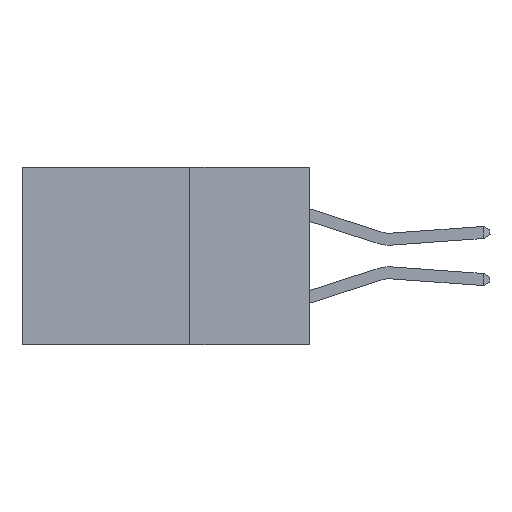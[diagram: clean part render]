
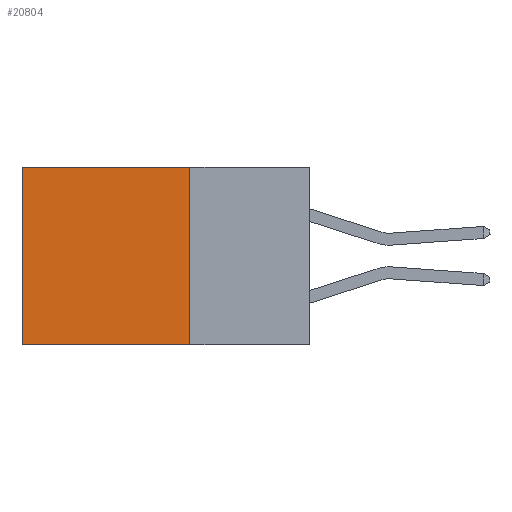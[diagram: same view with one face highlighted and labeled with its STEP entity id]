
A CAD part, left-side view. The second image highlights one B-rep face of the part: STEP entity #20804.
In plain terms, the highlighted planar face has unit normal (-1, 0, 0).
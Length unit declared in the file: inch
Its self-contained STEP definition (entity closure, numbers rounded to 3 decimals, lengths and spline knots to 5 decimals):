
#296 = EDGE_CURVE ( 'NONE', #18656, #12175, #3849, .T. ) ;
#745 = DIRECTION ( 'NONE',  ( 1., 0., 0. ) ) ;
#1654 = LINE ( 'NONE', #13209, #6766 ) ;
#2615 = DIRECTION ( 'NONE',  ( 0., 0., -1. ) ) ;
#3567 = ORIENTED_EDGE ( 'NONE', *, *, #8030, .F. ) ;
#3749 = VERTEX_POINT ( 'NONE', #14602 ) ;
#3849 = LINE ( 'NONE', #6229, #22401 ) ;
#5261 = FACE_OUTER_BOUND ( 'NONE', #11096, .T. ) ;
#6229 = CARTESIAN_POINT ( 'NONE',  ( 0.298, 0.6, 0. ) ) ;
#6607 = DIRECTION ( 'NONE',  ( 0., 0., -1. ) ) ;
#6766 = VECTOR ( 'NONE', #7160, 39.37008 ) ;
#7160 = DIRECTION ( 'NONE',  ( 0., 1., 0. ) ) ;
#7564 = VECTOR ( 'NONE', #18935, 39.37008 ) ;
#8030 = EDGE_CURVE ( 'NONE', #23668, #3749, #8172, .T. ) ;
#8172 = LINE ( 'NONE', #16945, #7564 ) ;
#9909 = ORIENTED_EDGE ( 'NONE', *, *, #16165, .T. ) ;
#10617 = CARTESIAN_POINT ( 'NONE',  ( 0.298, 0.25, -0.37 ) ) ;
#11096 = EDGE_LOOP ( 'NONE', ( #12236, #18182, #3567, #9909 ) ) ;
#11185 = EDGE_CURVE ( 'NONE', #3749, #12175, #22344, .T. ) ;
#11545 = AXIS2_PLACEMENT_3D ( 'NONE', #21764, #745, #6607 ) ;
#11629 = VECTOR ( 'NONE', #14143, 39.37008 ) ;
#12175 = VERTEX_POINT ( 'NONE', #22832 ) ;
#12236 = ORIENTED_EDGE ( 'NONE', *, *, #296, .T. ) ;
#13209 = CARTESIAN_POINT ( 'NONE',  ( 0.298, 0.25, 0. ) ) ;
#14143 = DIRECTION ( 'NONE',  ( 0., 1., 0. ) ) ;
#14602 = CARTESIAN_POINT ( 'NONE',  ( 0.298, 0.25, -0.37 ) ) ;
#15322 = CARTESIAN_POINT ( 'NONE',  ( 0.298, 0.6, 0. ) ) ;
#15514 = CARTESIAN_POINT ( 'NONE',  ( 0.298, 0.25, 0. ) ) ;
#16165 = EDGE_CURVE ( 'NONE', #23668, #18656, #1654, .T. ) ;
#16945 = CARTESIAN_POINT ( 'NONE',  ( 0.298, 0.25, 0. ) ) ;
#18182 = ORIENTED_EDGE ( 'NONE', *, *, #11185, .F. ) ;
#18656 = VERTEX_POINT ( 'NONE', #15322 ) ;
#18935 = DIRECTION ( 'NONE',  ( 0., 0., -1. ) ) ;
#19876 = PLANE ( 'NONE',  #11545 ) ;
#20804 = ADVANCED_FACE ( 'NONE', ( #5261 ), #19876, .F. ) ;
#21764 = CARTESIAN_POINT ( 'NONE',  ( 0.298, 0.25, 0. ) ) ;
#22344 = LINE ( 'NONE', #10617, #11629 ) ;
#22401 = VECTOR ( 'NONE', #2615, 39.37008 ) ;
#22832 = CARTESIAN_POINT ( 'NONE',  ( 0.298, 0.6, -0.37 ) ) ;
#23668 = VERTEX_POINT ( 'NONE', #15514 ) ;
